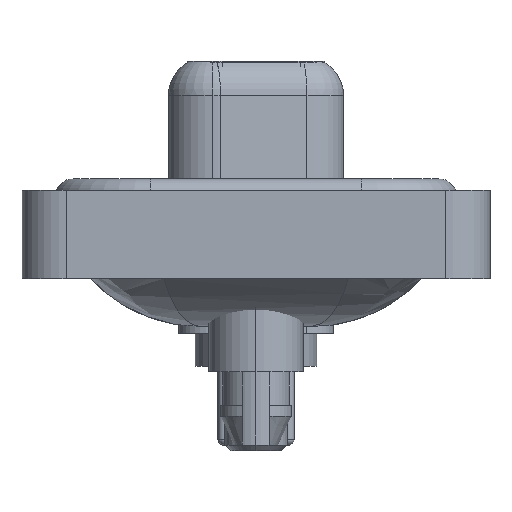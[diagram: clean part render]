
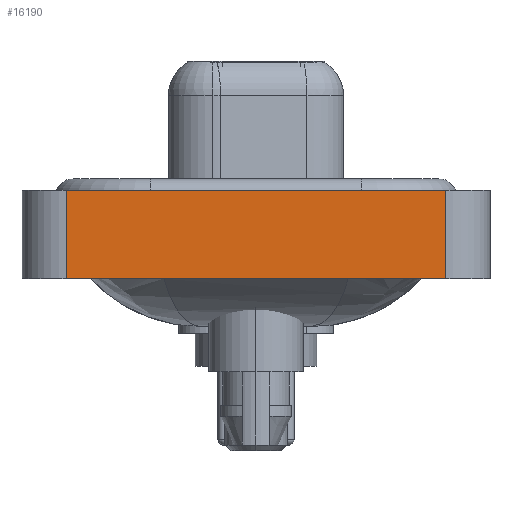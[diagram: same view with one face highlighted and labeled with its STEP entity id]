
A CAD part, left-side view. The second image highlights one B-rep face of the part: STEP entity #16190.
In plain terms, the highlighted planar face has unit normal (-1, 0, 0).
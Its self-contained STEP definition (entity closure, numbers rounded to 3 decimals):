
#784 = VERTEX_POINT ( 'NONE', #13861 ) ;
#2742 = CARTESIAN_POINT ( 'NONE',  ( -7.35, -8.55, 0.4 ) ) ;
#2989 = CARTESIAN_POINT ( 'NONE',  ( -7.35, -8.55, 0.4 ) ) ;
#3512 = VECTOR ( 'NONE', #7282, 1000. ) ;
#3694 = VERTEX_POINT ( 'NONE', #20178 ) ;
#5272 = DIRECTION ( 'NONE',  ( 0., 0., 1. ) ) ;
#5320 = CARTESIAN_POINT ( 'NONE',  ( -7.35, 8.55, -3.6 ) ) ;
#5629 = VERTEX_POINT ( 'NONE', #2742 ) ;
#7045 = CARTESIAN_POINT ( 'NONE',  ( -7.35, -8.55, -3.6 ) ) ;
#7282 = DIRECTION ( 'NONE',  ( 0., 0., 1. ) ) ;
#7413 = AXIS2_PLACEMENT_3D ( 'NONE', #19723, #19849, #23155 ) ;
#8023 = ORIENTED_EDGE ( 'NONE', *, *, #9866, .F. ) ;
#9067 = FACE_OUTER_BOUND ( 'NONE', #16006, .T. ) ;
#9178 = VECTOR ( 'NONE', #19544, 1000. ) ;
#9416 = ORIENTED_EDGE ( 'NONE', *, *, #21279, .F. ) ;
#9751 = ORIENTED_EDGE ( 'NONE', *, *, #20890, .T. ) ;
#9866 = EDGE_CURVE ( 'NONE', #3694, #5629, #21210, .T. ) ;
#10203 = DIRECTION ( 'NONE',  ( 0., -1., 0. ) ) ;
#12493 = PLANE ( 'NONE',  #7413 ) ;
#13335 = VECTOR ( 'NONE', #5272, 1000. ) ;
#13861 = CARTESIAN_POINT ( 'NONE',  ( -7.35, -8.55, -3.6 ) ) ;
#16006 = EDGE_LOOP ( 'NONE', ( #18697, #8023, #9416, #9751 ) ) ;
#16190 = ADVANCED_FACE ( 'NONE', ( #9067 ), #12493, .T. ) ;
#17428 = EDGE_CURVE ( 'NONE', #784, #5629, #21501, .T. ) ;
#17867 = VECTOR ( 'NONE', #10203, 1000. ) ;
#18697 = ORIENTED_EDGE ( 'NONE', *, *, #17428, .T. ) ;
#19266 = CARTESIAN_POINT ( 'NONE',  ( -7.35, 8.55, -3.6 ) ) ;
#19544 = DIRECTION ( 'NONE',  ( 0., -1., 0. ) ) ;
#19723 = CARTESIAN_POINT ( 'NONE',  ( -7.35, -8.55, -3.6 ) ) ;
#19849 = DIRECTION ( 'NONE',  ( -1., 0., 0. ) ) ;
#20024 = VERTEX_POINT ( 'NONE', #5320 ) ;
#20178 = CARTESIAN_POINT ( 'NONE',  ( -7.35, 8.55, 0.4 ) ) ;
#20890 = EDGE_CURVE ( 'NONE', #20024, #784, #21421, .T. ) ;
#21210 = LINE ( 'NONE', #2989, #17867 ) ;
#21279 = EDGE_CURVE ( 'NONE', #20024, #3694, #23048, .T. ) ;
#21421 = LINE ( 'NONE', #23432, #9178 ) ;
#21501 = LINE ( 'NONE', #7045, #3512 ) ;
#23048 = LINE ( 'NONE', #19266, #13335 ) ;
#23155 = DIRECTION ( 'NONE',  ( 0., 0., 1. ) ) ;
#23432 = CARTESIAN_POINT ( 'NONE',  ( -7.35, -8.55, -3.6 ) ) ;
